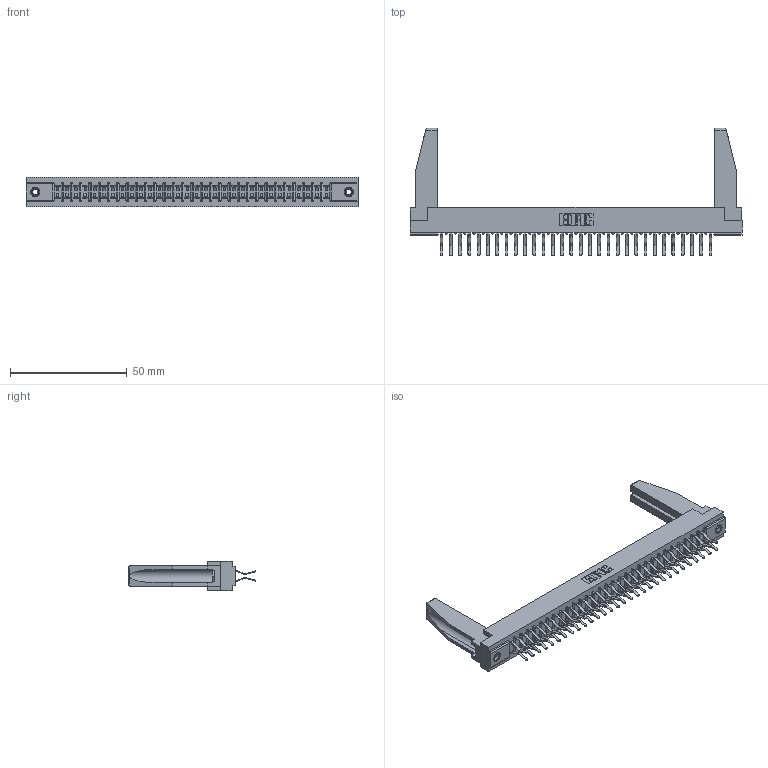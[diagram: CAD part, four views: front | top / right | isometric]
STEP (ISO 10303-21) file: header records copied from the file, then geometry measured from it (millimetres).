
FILE_DESCRIPTION (( 'STEP AP203' ), '1' );
FILE_NAME ('307-060-560-278.STEP', '2019-09-06T15:49:04', ( '' ), ( '' ), 'SwSTEP 2.0', 'SolidWorks 2016', '' );
FILE_SCHEMA (( 'CONFIG_CONTROL_DESIGN' ));
Length unit declared in the file: inch
Products named in the file (5): 345-250-001_345-250-001-102; 307-060-560-278; 307-290-001_560; 307 Part_.156 Dia Mounting Holes; 307-220-078
Assembly tree (65 placements, depth 2):
  307-060-560-278
    307 Part_.156 Dia Mounting Holes
    307-290-001_560  x60
    307-220-078  x2
    345-250-001_345-250-001-102  x2
Bounding box: 141.88 x 54.43 x 12.7 mm (x, y, z)
Volume: 19070.8 mm3; surface area: 22435.1 mm2
Topology: 65 solids, 65 shells, 3279 faces, 9173 edges, 5942 vertices
Faces by surface type: plane 2134, cylinder 1067, sphere 62, cone 12, torus 4
Entity records: 30701 total; most frequent: CARTESIAN_POINT 5036, ORIENTED_EDGE 4948, DIRECTION 4892, EDGE_CURVE 2474, VECTOR 1896, LINE 1896, VERTEX_POINT 1600, AXIS2_PLACEMENT_3D 1498
